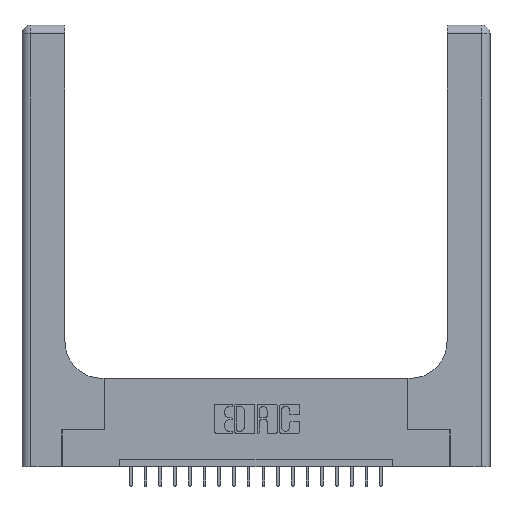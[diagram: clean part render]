
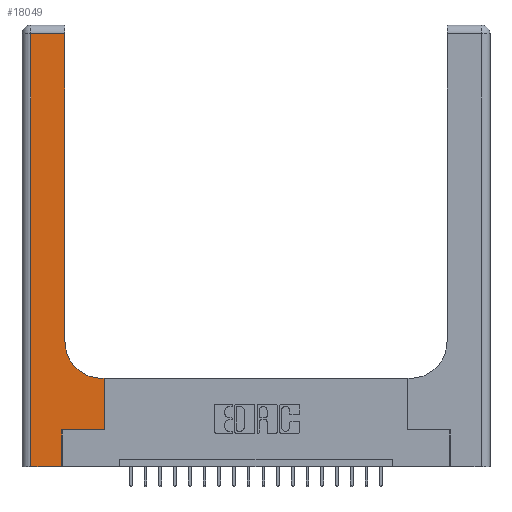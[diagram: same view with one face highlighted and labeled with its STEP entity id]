
A CAD part, top view. The second image highlights one B-rep face of the part: STEP entity #18049.
In plain terms, the highlighted planar face has unit normal (0, 0, 1).
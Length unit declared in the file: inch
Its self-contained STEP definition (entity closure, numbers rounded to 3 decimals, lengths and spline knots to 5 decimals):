
#177 = DIRECTION ( 'NONE',  ( 0., 1., 0. ) ) ;
#342 = DIRECTION ( 'NONE',  ( -1., 0., 0. ) ) ;
#355 = CARTESIAN_POINT ( 'NONE',  ( 0.5585, 0.6, 0.37 ) ) ;
#699 = EDGE_CURVE ( 'NONE', #17999, #16349, #4458, .T. ) ;
#725 = LINE ( 'NONE', #21367, #8915 ) ;
#910 = DIRECTION ( 'NONE',  ( 1., 0., 0. ) ) ;
#1332 = LINE ( 'NONE', #20088, #1428 ) ;
#1428 = VECTOR ( 'NONE', #910, 39.37008 ) ;
#1457 = DIRECTION ( 'NONE',  ( 0., 0., -1. ) ) ;
#1560 = EDGE_CURVE ( 'NONE', #4902, #12941, #725, .T. ) ;
#2372 = VERTEX_POINT ( 'NONE', #12831 ) ;
#2668 = DIRECTION ( 'NONE',  ( 1., 0., 0. ) ) ;
#4029 = ORIENTED_EDGE ( 'NONE', *, *, #1560, .T. ) ;
#4458 = LINE ( 'NONE', #21732, #15690 ) ;
#4722 = ORIENTED_EDGE ( 'NONE', *, *, #15344, .T. ) ;
#4770 = ORIENTED_EDGE ( 'NONE', *, *, #6292, .T. ) ;
#4902 = VERTEX_POINT ( 'NONE', #355 ) ;
#5140 = FACE_OUTER_BOUND ( 'NONE', #13863, .T. ) ;
#5724 = DIRECTION ( 'NONE',  ( 0., 1., 0. ) ) ;
#6100 = ORIENTED_EDGE ( 'NONE', *, *, #699, .T. ) ;
#6292 = EDGE_CURVE ( 'NONE', #9321, #13835, #9818, .T. ) ;
#7013 = EDGE_CURVE ( 'NONE', #13835, #17999, #19581, .T. ) ;
#7301 = VECTOR ( 'NONE', #177, 39.37008 ) ;
#7511 = CARTESIAN_POINT ( 'NONE',  ( 0.2915, 2.94, 0.37 ) ) ;
#7540 = DIRECTION ( 'NONE',  ( -1., 0., 0. ) ) ;
#8570 = CIRCLE ( 'NONE', #16777, 0.25 ) ;
#8907 = EDGE_CURVE ( 'NONE', #16349, #2372, #14534, .T. ) ;
#8915 = VECTOR ( 'NONE', #11005, 39.37008 ) ;
#9181 = LINE ( 'NONE', #17460, #13199 ) ;
#9321 = VERTEX_POINT ( 'NONE', #19622 ) ;
#9456 = VECTOR ( 'NONE', #12034, 39.37008 ) ;
#9818 = LINE ( 'NONE', #15603, #7301 ) ;
#9856 = EDGE_CURVE ( 'NONE', #12941, #9321, #8570, .T. ) ;
#9881 = ORIENTED_EDGE ( 'NONE', *, *, #7013, .T. ) ;
#9965 = ORIENTED_EDGE ( 'NONE', *, *, #9856, .T. ) ;
#10167 = CARTESIAN_POINT ( 'NONE',  ( 0., 3., 0.37 ) ) ;
#10240 = CARTESIAN_POINT ( 'NONE',  ( 0.269, 0., 0.37 ) ) ;
#10428 = CARTESIAN_POINT ( 'NONE',  ( 0.06, 0., 0.37 ) ) ;
#11005 = DIRECTION ( 'NONE',  ( -1., 0., 0. ) ) ;
#11434 = ORIENTED_EDGE ( 'NONE', *, *, #8907, .T. ) ;
#12034 = DIRECTION ( 'NONE',  ( 0., 1., 0. ) ) ;
#12493 = EDGE_CURVE ( 'NONE', #17636, #4902, #9181, .T. ) ;
#12831 = CARTESIAN_POINT ( 'NONE',  ( 0.269, 0., 0.37 ) ) ;
#12941 = VERTEX_POINT ( 'NONE', #14068 ) ;
#13199 = VECTOR ( 'NONE', #5724, 39.37008 ) ;
#13523 = ORIENTED_EDGE ( 'NONE', *, *, #19003, .T. ) ;
#13744 = CARTESIAN_POINT ( 'NONE',  ( 0.06, 2.94, 0.37 ) ) ;
#13810 = VECTOR ( 'NONE', #2668, 39.37008 ) ;
#13835 = VERTEX_POINT ( 'NONE', #7511 ) ;
#13863 = EDGE_LOOP ( 'NONE', ( #4770, #9881, #6100, #11434, #13523, #4722, #15021, #4029, #9965 ) ) ;
#13922 = LINE ( 'NONE', #10240, #9456 ) ;
#14068 = CARTESIAN_POINT ( 'NONE',  ( 0.5415, 0.6, 0.37 ) ) ;
#14466 = CARTESIAN_POINT ( 'NONE',  ( 0., 2.94, 0.37 ) ) ;
#14534 = LINE ( 'NONE', #17981, #13810 ) ;
#15021 = ORIENTED_EDGE ( 'NONE', *, *, #12493, .T. ) ;
#15308 = PLANE ( 'NONE',  #21526 ) ;
#15344 = EDGE_CURVE ( 'NONE', #19774, #17636, #1332, .T. ) ;
#15603 = CARTESIAN_POINT ( 'NONE',  ( 0.2915, 3., 0.37 ) ) ;
#15690 = VECTOR ( 'NONE', #17870, 39.37008 ) ;
#16349 = VERTEX_POINT ( 'NONE', #10428 ) ;
#16771 = CARTESIAN_POINT ( 'NONE',  ( 0.5415, 0.85, 0.37 ) ) ;
#16777 = AXIS2_PLACEMENT_3D ( 'NONE', #16771, #1457, #20219 ) ;
#17238 = CARTESIAN_POINT ( 'NONE',  ( 0.5585, 0.25, 0.37 ) ) ;
#17460 = CARTESIAN_POINT ( 'NONE',  ( 0.5585, 0.25, 0.37 ) ) ;
#17636 = VERTEX_POINT ( 'NONE', #17238 ) ;
#17689 = VECTOR ( 'NONE', #7540, 39.37008 ) ;
#17870 = DIRECTION ( 'NONE',  ( 0., -1., 0. ) ) ;
#17981 = CARTESIAN_POINT ( 'NONE',  ( 0., 0., 0.37 ) ) ;
#17999 = VERTEX_POINT ( 'NONE', #13744 ) ;
#18049 = ADVANCED_FACE ( 'NONE', ( #5140 ), #15308, .F. ) ;
#19003 = EDGE_CURVE ( 'NONE', #2372, #19774, #13922, .T. ) ;
#19581 = LINE ( 'NONE', #14466, #17689 ) ;
#19622 = CARTESIAN_POINT ( 'NONE',  ( 0.2915, 0.85, 0.37 ) ) ;
#19774 = VERTEX_POINT ( 'NONE', #21750 ) ;
#20088 = CARTESIAN_POINT ( 'NONE',  ( 0.269, 0.25, 0.37 ) ) ;
#20219 = DIRECTION ( 'NONE',  ( 1., 0., 0. ) ) ;
#20650 = DIRECTION ( 'NONE',  ( 0., 0., -1. ) ) ;
#21367 = CARTESIAN_POINT ( 'NONE',  ( 0.2915, 0.6, 0.37 ) ) ;
#21526 = AXIS2_PLACEMENT_3D ( 'NONE', #10167, #20650, #342 ) ;
#21732 = CARTESIAN_POINT ( 'NONE',  ( 0.06, 3., 0.37 ) ) ;
#21750 = CARTESIAN_POINT ( 'NONE',  ( 0.269, 0.25, 0.37 ) ) ;
